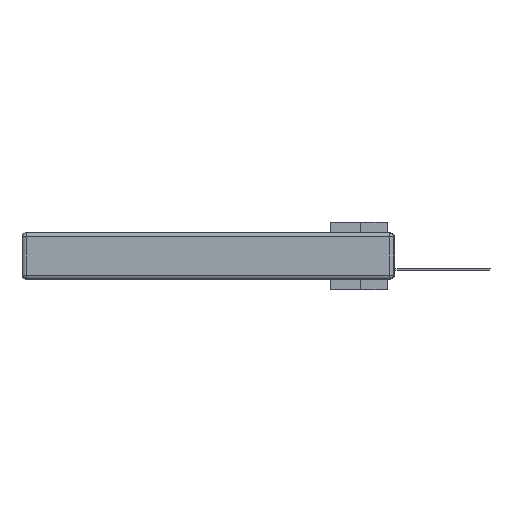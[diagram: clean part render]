
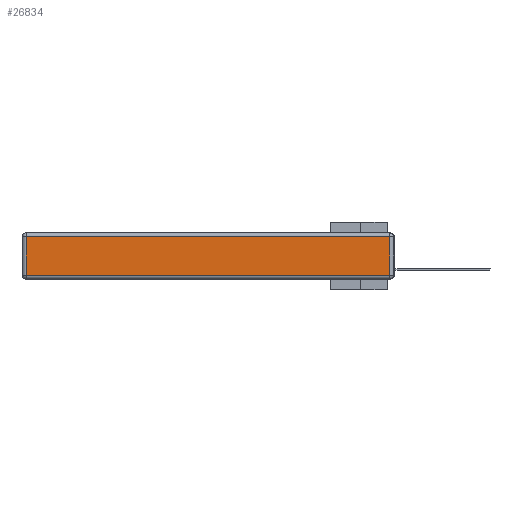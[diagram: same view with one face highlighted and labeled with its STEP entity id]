
A CAD part, left-side view. The second image highlights one B-rep face of the part: STEP entity #26834.
In plain terms, the highlighted planar face has unit normal (-1, 0, 0).
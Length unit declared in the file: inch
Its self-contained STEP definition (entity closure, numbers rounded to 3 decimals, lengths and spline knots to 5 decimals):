
#2799 = VECTOR ( 'NONE', #19496, 39.37008 ) ;
#5525 = VERTEX_POINT ( 'NONE', #7732 ) ;
#7260 = CARTESIAN_POINT ( 'NONE',  ( 0., 0., -0.313 ) ) ;
#7732 = CARTESIAN_POINT ( 'NONE',  ( 0., 0.03, -0.03 ) ) ;
#8649 = DIRECTION ( 'NONE',  ( 0., 0., 1. ) ) ;
#10126 = VERTEX_POINT ( 'NONE', #32588 ) ;
#10571 = AXIS2_PLACEMENT_3D ( 'NONE', #14938, #33073, #8649 ) ;
#12072 = VECTOR ( 'NONE', #14923, 39.37008 ) ;
#13558 = LINE ( 'NONE', #19694, #20802 ) ;
#13944 = ORIENTED_EDGE ( 'NONE', *, *, #30784, .T. ) ;
#14923 = DIRECTION ( 'NONE',  ( 0., 0., -1. ) ) ;
#14938 = CARTESIAN_POINT ( 'NONE',  ( 0., 0., -0.343 ) ) ;
#18021 = CARTESIAN_POINT ( 'NONE',  ( 0., 2.72, -0.343 ) ) ;
#18357 = CARTESIAN_POINT ( 'NONE',  ( 0., 2.72, -0.313 ) ) ;
#19496 = DIRECTION ( 'NONE',  ( 0., -1., 0. ) ) ;
#19694 = CARTESIAN_POINT ( 'NONE',  ( 0., 0.03, -0.343 ) ) ;
#20572 = LINE ( 'NONE', #23589, #26872 ) ;
#20802 = VECTOR ( 'NONE', #38557, 39.37008 ) ;
#22499 = FACE_OUTER_BOUND ( 'NONE', #27814, .T. ) ;
#22542 = VERTEX_POINT ( 'NONE', #18357 ) ;
#22992 = ORIENTED_EDGE ( 'NONE', *, *, #30198, .T. ) ;
#23589 = CARTESIAN_POINT ( 'NONE',  ( 0., 2.75, -0.03 ) ) ;
#25051 = ORIENTED_EDGE ( 'NONE', *, *, #33471, .T. ) ;
#26834 = ADVANCED_FACE ( 'NONE', ( #22499 ), #33343, .T. ) ;
#26872 = VECTOR ( 'NONE', #40118, 39.37008 ) ;
#27601 = LINE ( 'NONE', #18021, #12072 ) ;
#27654 = VERTEX_POINT ( 'NONE', #38827 ) ;
#27814 = EDGE_LOOP ( 'NONE', ( #13944, #38533, #25051, #22992 ) ) ;
#30198 = EDGE_CURVE ( 'NONE', #27654, #22542, #27601, .T. ) ;
#30784 = EDGE_CURVE ( 'NONE', #22542, #10126, #34322, .T. ) ;
#32588 = CARTESIAN_POINT ( 'NONE',  ( 0., 0.03, -0.313 ) ) ;
#33073 = DIRECTION ( 'NONE',  ( -1., 0., 0. ) ) ;
#33343 = PLANE ( 'NONE',  #10571 ) ;
#33471 = EDGE_CURVE ( 'NONE', #5525, #27654, #20572, .T. ) ;
#34322 = LINE ( 'NONE', #7260, #2799 ) ;
#36185 = EDGE_CURVE ( 'NONE', #10126, #5525, #13558, .T. ) ;
#38533 = ORIENTED_EDGE ( 'NONE', *, *, #36185, .T. ) ;
#38557 = DIRECTION ( 'NONE',  ( 0., 0., 1. ) ) ;
#38827 = CARTESIAN_POINT ( 'NONE',  ( 0., 2.72, -0.03 ) ) ;
#40118 = DIRECTION ( 'NONE',  ( 0., 1., 0. ) ) ;
